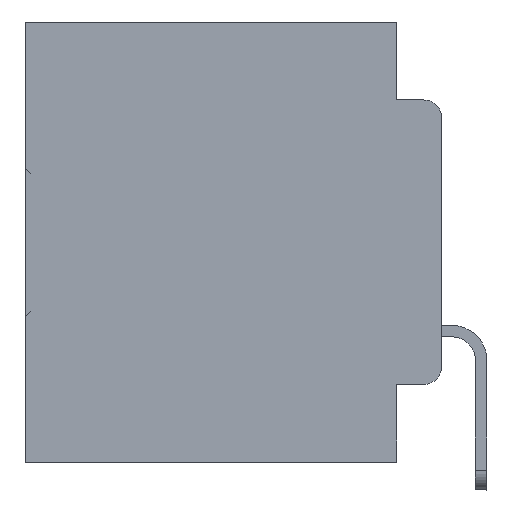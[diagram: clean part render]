
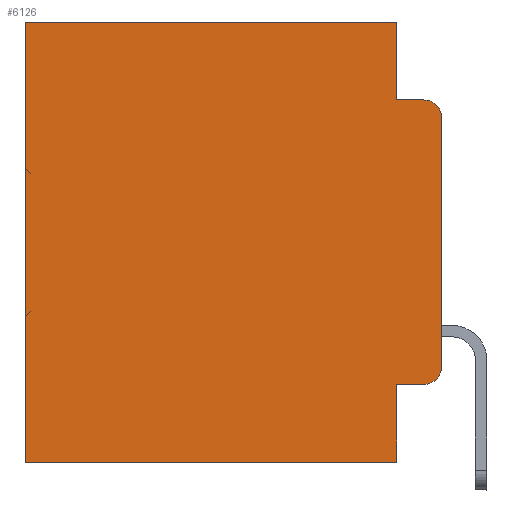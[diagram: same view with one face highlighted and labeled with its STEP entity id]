
A CAD part, left-side view. The second image highlights one B-rep face of the part: STEP entity #6126.
In plain terms, the highlighted planar face has unit normal (-1, 0, 0).
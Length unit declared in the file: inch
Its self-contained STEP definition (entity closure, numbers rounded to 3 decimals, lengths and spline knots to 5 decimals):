
#280 = CARTESIAN_POINT ( 'NONE',  ( 0.298, 0.02, -0.3915 ) ) ;
#383 = LINE ( 'NONE', #12396, #20796 ) ;
#857 = VERTEX_POINT ( 'NONE', #26510 ) ;
#1616 = EDGE_CURVE ( 'NONE', #28005, #2630, #11586, .T. ) ;
#1658 = VECTOR ( 'NONE', #11950, 39.37008 ) ;
#2586 = ORIENTED_EDGE ( 'NONE', *, *, #23670, .F. ) ;
#2630 = VERTEX_POINT ( 'NONE', #31485 ) ;
#3881 = DIRECTION ( 'NONE',  ( 0., 0., -1. ) ) ;
#4197 = EDGE_CURVE ( 'NONE', #30574, #28005, #8221, .T. ) ;
#4310 = VECTOR ( 'NONE', #5334, 39.37008 ) ;
#5002 = AXIS2_PLACEMENT_3D ( 'NONE', #9659, #29084, #3881 ) ;
#5334 = DIRECTION ( 'NONE',  ( 0., -1., 0. ) ) ;
#6126 = ADVANCED_FACE ( 'NONE', ( #30959 ), #19419, .F. ) ;
#6143 = VERTEX_POINT ( 'NONE', #24954 ) ;
#6210 = CARTESIAN_POINT ( 'NONE',  ( 0.298, 0., -0.1085 ) ) ;
#6634 = VERTEX_POINT ( 'NONE', #21371 ) ;
#6878 = CARTESIAN_POINT ( 'NONE',  ( 0.298, 0., 0. ) ) ;
#7260 = DIRECTION ( 'NONE',  ( 0., 1., 0. ) ) ;
#7371 = DIRECTION ( 'NONE',  ( 0., 0., -1. ) ) ;
#8221 = LINE ( 'NONE', #30679, #35083 ) ;
#8851 = EDGE_CURVE ( 'NONE', #6143, #6634, #19984, .T. ) ;
#9020 = EDGE_CURVE ( 'NONE', #857, #34444, #19953, .T. ) ;
#9178 = CARTESIAN_POINT ( 'NONE',  ( 0.298, 0., -0.5 ) ) ;
#9659 = CARTESIAN_POINT ( 'NONE',  ( 0.298, 0.02, -0.1085 ) ) ;
#9912 = ORIENTED_EDGE ( 'NONE', *, *, #31091, .F. ) ;
#9974 = ORIENTED_EDGE ( 'NONE', *, *, #4197, .F. ) ;
#10162 = VERTEX_POINT ( 'NONE', #6210 ) ;
#10908 = DIRECTION ( 'NONE',  ( -1., 0., 0. ) ) ;
#11004 = ORIENTED_EDGE ( 'NONE', *, *, #9020, .F. ) ;
#11017 = DIRECTION ( 'NONE',  ( 0., 0., -1. ) ) ;
#11043 = EDGE_CURVE ( 'NONE', #30574, #11654, #30667, .T. ) ;
#11586 = LINE ( 'NONE', #29932, #4310 ) ;
#11654 = VERTEX_POINT ( 'NONE', #21437 ) ;
#11950 = DIRECTION ( 'NONE',  ( 0., 0., -1. ) ) ;
#12063 = EDGE_LOOP ( 'NONE', ( #9912, #28679, #28121, #9974, #35356, #34343, #11004, #2586, #31941, #30311 ) ) ;
#12396 = CARTESIAN_POINT ( 'NONE',  ( 0.298, 0.051, 0. ) ) ;
#12669 = EDGE_CURVE ( 'NONE', #28081, #6143, #20159, .T. ) ;
#13777 = AXIS2_PLACEMENT_3D ( 'NONE', #33300, #27966, #22224 ) ;
#15943 = EDGE_CURVE ( 'NONE', #11654, #34444, #19848, .T. ) ;
#17058 = DIRECTION ( 'NONE',  ( 0., 1., 0. ) ) ;
#17297 = CARTESIAN_POINT ( 'NONE',  ( 0.298, 0.051, -0.0885 ) ) ;
#19419 = PLANE ( 'NONE',  #13777 ) ;
#19729 = CARTESIAN_POINT ( 'NONE',  ( 0.298, 0.051, 0. ) ) ;
#19848 = LINE ( 'NONE', #28585, #1658 ) ;
#19953 = LINE ( 'NONE', #9178, #22195 ) ;
#19984 = CIRCLE ( 'NONE', #31708, 0.02 ) ;
#20159 = LINE ( 'NONE', #21837, #28816 ) ;
#20796 = VECTOR ( 'NONE', #7371, 39.37008 ) ;
#21346 = DIRECTION ( 'NONE',  ( 0., -1., 0. ) ) ;
#21371 = CARTESIAN_POINT ( 'NONE',  ( 0.298, 0., -0.3915 ) ) ;
#21437 = CARTESIAN_POINT ( 'NONE',  ( 0.298, 0.473, 0. ) ) ;
#21837 = CARTESIAN_POINT ( 'NONE',  ( 0.298, 0.051, -0.4115 ) ) ;
#22110 = VECTOR ( 'NONE', #7260, 39.37008 ) ;
#22195 = VECTOR ( 'NONE', #17058, 39.37008 ) ;
#22224 = DIRECTION ( 'NONE',  ( 0., 0., -1. ) ) ;
#23670 = EDGE_CURVE ( 'NONE', #28081, #857, #383, .T. ) ;
#24349 = CARTESIAN_POINT ( 'NONE',  ( 0.298, 0., 0. ) ) ;
#24761 = CARTESIAN_POINT ( 'NONE',  ( 0.298, 0.051, -0.4115 ) ) ;
#24941 = CIRCLE ( 'NONE', #5002, 0.02 ) ;
#24954 = CARTESIAN_POINT ( 'NONE',  ( 0.298, 0.02, -0.4115 ) ) ;
#25727 = CARTESIAN_POINT ( 'NONE',  ( 0.298, 0.473, -0.5 ) ) ;
#26211 = VECTOR ( 'NONE', #30032, 39.37008 ) ;
#26510 = CARTESIAN_POINT ( 'NONE',  ( 0.298, 0.051, -0.5 ) ) ;
#27966 = DIRECTION ( 'NONE',  ( 1., 0., 0. ) ) ;
#28005 = VERTEX_POINT ( 'NONE', #17297 ) ;
#28081 = VERTEX_POINT ( 'NONE', #24761 ) ;
#28121 = ORIENTED_EDGE ( 'NONE', *, *, #1616, .F. ) ;
#28585 = CARTESIAN_POINT ( 'NONE',  ( 0.298, 0.473, 0. ) ) ;
#28679 = ORIENTED_EDGE ( 'NONE', *, *, #33850, .T. ) ;
#28816 = VECTOR ( 'NONE', #21346, 39.37008 ) ;
#29084 = DIRECTION ( 'NONE',  ( -1., 0., 0. ) ) ;
#29932 = CARTESIAN_POINT ( 'NONE',  ( 0.298, 0.051, -0.0885 ) ) ;
#30032 = DIRECTION ( 'NONE',  ( 0., 0., -1. ) ) ;
#30311 = ORIENTED_EDGE ( 'NONE', *, *, #8851, .T. ) ;
#30574 = VERTEX_POINT ( 'NONE', #19729 ) ;
#30667 = LINE ( 'NONE', #6878, #22110 ) ;
#30679 = CARTESIAN_POINT ( 'NONE',  ( 0.298, 0.051, 0. ) ) ;
#30959 = FACE_OUTER_BOUND ( 'NONE', #12063, .T. ) ;
#31091 = EDGE_CURVE ( 'NONE', #10162, #6634, #34409, .T. ) ;
#31151 = DIRECTION ( 'NONE',  ( 0., 0., -1. ) ) ;
#31485 = CARTESIAN_POINT ( 'NONE',  ( 0.298, 0.02, -0.0885 ) ) ;
#31708 = AXIS2_PLACEMENT_3D ( 'NONE', #280, #10908, #11017 ) ;
#31941 = ORIENTED_EDGE ( 'NONE', *, *, #12669, .T. ) ;
#33300 = CARTESIAN_POINT ( 'NONE',  ( 0.298, 0., 0. ) ) ;
#33850 = EDGE_CURVE ( 'NONE', #10162, #2630, #24941, .T. ) ;
#34343 = ORIENTED_EDGE ( 'NONE', *, *, #15943, .T. ) ;
#34409 = LINE ( 'NONE', #24349, #26211 ) ;
#34444 = VERTEX_POINT ( 'NONE', #25727 ) ;
#35083 = VECTOR ( 'NONE', #31151, 39.37008 ) ;
#35356 = ORIENTED_EDGE ( 'NONE', *, *, #11043, .T. ) ;
